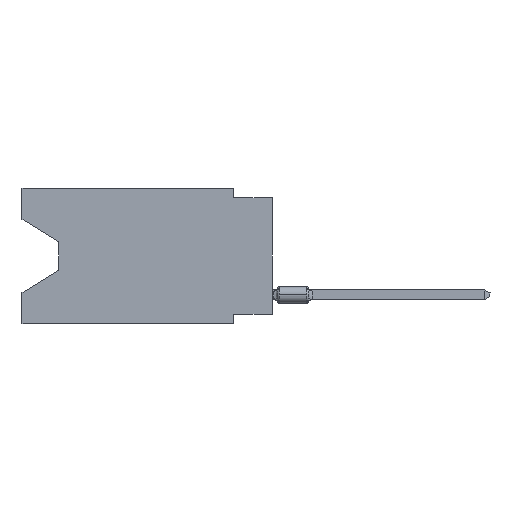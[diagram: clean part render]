
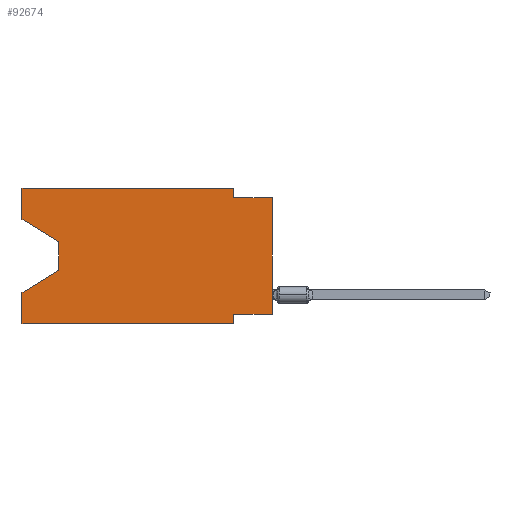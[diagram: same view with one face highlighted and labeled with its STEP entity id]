
A CAD part, left-side view. The second image highlights one B-rep face of the part: STEP entity #92674.
In plain terms, the highlighted planar face has unit normal (-1, 0, 0).
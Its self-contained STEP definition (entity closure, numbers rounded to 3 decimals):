
#936 = LINE ( 'NONE', #16467, #38794 ) ;
#3930 = DIRECTION ( 'NONE',  ( 0., -1., 0. ) ) ;
#4778 = ORIENTED_EDGE ( 'NONE', *, *, #99260, .F. ) ;
#4803 = EDGE_LOOP ( 'NONE', ( #96292, #86829, #64550, #33960, #16881, #38599, #81066, #36115, #4778, #14226, #68435, #78294 ) ) ;
#5382 = CARTESIAN_POINT ( 'NONE',  ( 0., 13.97, -3.505 ) ) ;
#7507 = EDGE_CURVE ( 'NONE', #35727, #37396, #25123, .T. ) ;
#8821 = EDGE_CURVE ( 'NONE', #56160, #96466, #102596, .T. ) ;
#12257 = DIRECTION ( 'NONE',  ( 0., 0.855, -0.519 ) ) ;
#12744 = LINE ( 'NONE', #45912, #104707 ) ;
#12854 = VECTOR ( 'NONE', #44402, 1000. ) ;
#13930 = VECTOR ( 'NONE', #77529, 1000. ) ;
#14226 = ORIENTED_EDGE ( 'NONE', *, *, #32892, .F. ) ;
#15246 = LINE ( 'NONE', #81489, #44440 ) ;
#16467 = CARTESIAN_POINT ( 'NONE',  ( 0., 2.54, 0. ) ) ;
#16497 = VERTEX_POINT ( 'NONE', #46556 ) ;
#16881 = ORIENTED_EDGE ( 'NONE', *, *, #54284, .T. ) ;
#17884 = CARTESIAN_POINT ( 'NONE',  ( 0., 16.383, -6.852 ) ) ;
#18203 = CARTESIAN_POINT ( 'NONE',  ( 0., 16.383, -8.89 ) ) ;
#18759 = CARTESIAN_POINT ( 'NONE',  ( 0., 16.383, -2.038 ) ) ;
#20291 = DIRECTION ( 'NONE',  ( 0., 0., -1. ) ) ;
#20655 = VECTOR ( 'NONE', #55051, 1000. ) ;
#20692 = VERTEX_POINT ( 'NONE', #30276 ) ;
#21752 = PLANE ( 'NONE',  #35680 ) ;
#25123 = LINE ( 'NONE', #57755, #35064 ) ;
#27487 = LINE ( 'NONE', #44070, #68845 ) ;
#28313 = EDGE_CURVE ( 'NONE', #85619, #96466, #85705, .T. ) ;
#28381 = CARTESIAN_POINT ( 'NONE',  ( 0., 0., -0.635 ) ) ;
#30276 = CARTESIAN_POINT ( 'NONE',  ( 0., 2.54, -0.635 ) ) ;
#31796 = DIRECTION ( 'NONE',  ( 0., 0., 1. ) ) ;
#32892 = EDGE_CURVE ( 'NONE', #40037, #20692, #936, .T. ) ;
#33241 = VERTEX_POINT ( 'NONE', #71440 ) ;
#33960 = ORIENTED_EDGE ( 'NONE', *, *, #28313, .F. ) ;
#35064 = VECTOR ( 'NONE', #90363, 1000. ) ;
#35146 = CARTESIAN_POINT ( 'NONE',  ( 0., 2.54, 0. ) ) ;
#35680 = AXIS2_PLACEMENT_3D ( 'NONE', #38311, #55402, #102985 ) ;
#35727 = VERTEX_POINT ( 'NONE', #40829 ) ;
#36115 = ORIENTED_EDGE ( 'NONE', *, *, #55262, .T. ) ;
#37396 = VERTEX_POINT ( 'NONE', #42298 ) ;
#37784 = FACE_OUTER_BOUND ( 'NONE', #4803, .T. ) ;
#37981 = LINE ( 'NONE', #28381, #13930 ) ;
#38311 = CARTESIAN_POINT ( 'NONE',  ( 0., 16.383, 0. ) ) ;
#38599 = ORIENTED_EDGE ( 'NONE', *, *, #70441, .F. ) ;
#38794 = VECTOR ( 'NONE', #97723, 1000. ) ;
#40037 = VERTEX_POINT ( 'NONE', #35146 ) ;
#40829 = CARTESIAN_POINT ( 'NONE',  ( 0., 16.383, -2.038 ) ) ;
#42298 = CARTESIAN_POINT ( 'NONE',  ( 0., 16.383, 0. ) ) ;
#42724 = EDGE_CURVE ( 'NONE', #72935, #56160, #44360, .T. ) ;
#44070 = CARTESIAN_POINT ( 'NONE',  ( 0., 16.383, 0. ) ) ;
#44360 = LINE ( 'NONE', #53401, #98636 ) ;
#44402 = DIRECTION ( 'NONE',  ( 0., -0.855, -0.519 ) ) ;
#44440 = VECTOR ( 'NONE', #31796, 1000. ) ;
#45912 = CARTESIAN_POINT ( 'NONE',  ( 0., 0., -8.255 ) ) ;
#46556 = CARTESIAN_POINT ( 'NONE',  ( 0., 0., -0.635 ) ) ;
#47041 = LINE ( 'NONE', #79633, #20655 ) ;
#51884 = CARTESIAN_POINT ( 'NONE',  ( 0., 0., -8.255 ) ) ;
#52733 = CARTESIAN_POINT ( 'NONE',  ( 0., 13.97, -5.385 ) ) ;
#53401 = CARTESIAN_POINT ( 'NONE',  ( 0., 13.97, -3.505 ) ) ;
#53443 = LINE ( 'NONE', #18759, #12854 ) ;
#54284 = EDGE_CURVE ( 'NONE', #85619, #33241, #54547, .T. ) ;
#54547 = LINE ( 'NONE', #62562, #68245 ) ;
#55051 = DIRECTION ( 'NONE',  ( 0., 0., -1. ) ) ;
#55262 = EDGE_CURVE ( 'NONE', #86968, #16497, #15246, .T. ) ;
#55402 = DIRECTION ( 'NONE',  ( 1., 0., 0. ) ) ;
#56160 = VERTEX_POINT ( 'NONE', #52733 ) ;
#57755 = CARTESIAN_POINT ( 'NONE',  ( 0., 16.383, 0. ) ) ;
#59714 = EDGE_CURVE ( 'NONE', #37396, #40037, #27487, .T. ) ;
#60085 = EDGE_CURVE ( 'NONE', #86968, #97913, #12744, .T. ) ;
#60899 = DIRECTION ( 'NONE',  ( 0., 1., 0. ) ) ;
#62562 = CARTESIAN_POINT ( 'NONE',  ( 0., 16.383, -8.89 ) ) ;
#64550 = ORIENTED_EDGE ( 'NONE', *, *, #8821, .T. ) ;
#68245 = VECTOR ( 'NONE', #87660, 1000. ) ;
#68435 = ORIENTED_EDGE ( 'NONE', *, *, #59714, .F. ) ;
#68626 = DIRECTION ( 'NONE',  ( 0., 0., 1. ) ) ;
#68845 = VECTOR ( 'NONE', #3930, 1000. ) ;
#69466 = CARTESIAN_POINT ( 'NONE',  ( 0., 13.97, -5.385 ) ) ;
#70441 = EDGE_CURVE ( 'NONE', #97913, #33241, #47041, .T. ) ;
#70576 = VECTOR ( 'NONE', #68626, 1000. ) ;
#70718 = CARTESIAN_POINT ( 'NONE',  ( 0., 16.383, 0. ) ) ;
#71440 = CARTESIAN_POINT ( 'NONE',  ( 0., 2.54, -8.89 ) ) ;
#72935 = VERTEX_POINT ( 'NONE', #5382 ) ;
#76648 = VECTOR ( 'NONE', #12257, 1000. ) ;
#77529 = DIRECTION ( 'NONE',  ( 0., -1., 0. ) ) ;
#78294 = ORIENTED_EDGE ( 'NONE', *, *, #7507, .F. ) ;
#79633 = CARTESIAN_POINT ( 'NONE',  ( 0., 2.54, -8.89 ) ) ;
#81066 = ORIENTED_EDGE ( 'NONE', *, *, #60085, .F. ) ;
#81489 = CARTESIAN_POINT ( 'NONE',  ( 0., 0., 0. ) ) ;
#85619 = VERTEX_POINT ( 'NONE', #18203 ) ;
#85705 = LINE ( 'NONE', #70718, #70576 ) ;
#86829 = ORIENTED_EDGE ( 'NONE', *, *, #42724, .T. ) ;
#86944 = EDGE_CURVE ( 'NONE', #35727, #72935, #53443, .T. ) ;
#86968 = VERTEX_POINT ( 'NONE', #51884 ) ;
#87660 = DIRECTION ( 'NONE',  ( 0., -1., 0. ) ) ;
#90363 = DIRECTION ( 'NONE',  ( 0., 0., 1. ) ) ;
#92674 = ADVANCED_FACE ( 'NONE', ( #37784 ), #21752, .F. ) ;
#96292 = ORIENTED_EDGE ( 'NONE', *, *, #86944, .T. ) ;
#96466 = VERTEX_POINT ( 'NONE', #17884 ) ;
#97723 = DIRECTION ( 'NONE',  ( 0., 0., -1. ) ) ;
#97913 = VERTEX_POINT ( 'NONE', #103156 ) ;
#98636 = VECTOR ( 'NONE', #20291, 1000. ) ;
#99260 = EDGE_CURVE ( 'NONE', #20692, #16497, #37981, .T. ) ;
#102596 = LINE ( 'NONE', #69466, #76648 ) ;
#102985 = DIRECTION ( 'NONE',  ( 0., 0., -1. ) ) ;
#103156 = CARTESIAN_POINT ( 'NONE',  ( 0., 2.54, -8.255 ) ) ;
#104707 = VECTOR ( 'NONE', #60899, 1000. ) ;
